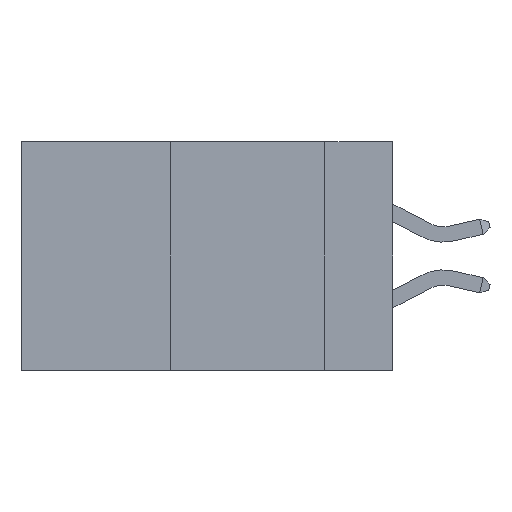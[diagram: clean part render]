
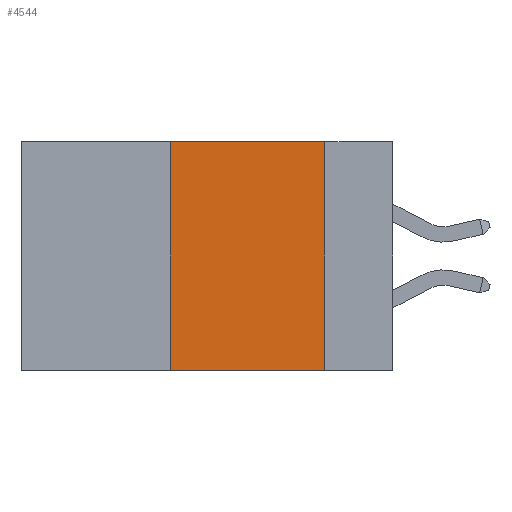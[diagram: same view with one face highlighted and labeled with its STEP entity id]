
A CAD part, left-side view. The second image highlights one B-rep face of the part: STEP entity #4544.
In plain terms, the highlighted planar face has unit normal (-1, 0, 0).
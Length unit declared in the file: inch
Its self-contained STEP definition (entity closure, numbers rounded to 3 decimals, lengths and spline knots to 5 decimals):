
#792 = DIRECTION ( 'NONE',  ( 0., 0., -1. ) ) ;
#850 = CARTESIAN_POINT ( 'NONE',  ( 0., 0.6, -0.37 ) ) ;
#1482 = CARTESIAN_POINT ( 'NONE',  ( 0., 0.6, 0. ) ) ;
#2125 = LINE ( 'NONE', #850, #16871 ) ;
#2255 = FACE_OUTER_BOUND ( 'NONE', #17594, .T. ) ;
#3643 = CARTESIAN_POINT ( 'NONE',  ( 0., 0.36, -0.37 ) ) ;
#4544 = ADVANCED_FACE ( 'NONE', ( #2255 ), #6492, .F. ) ;
#4695 = DIRECTION ( 'NONE',  ( 0., -1., 0. ) ) ;
#5399 = LINE ( 'NONE', #20824, #24518 ) ;
#5558 = VERTEX_POINT ( 'NONE', #3643 ) ;
#6116 = EDGE_CURVE ( 'NONE', #16704, #19668, #18142, .T. ) ;
#6232 = ORIENTED_EDGE ( 'NONE', *, *, #14198, .F. ) ;
#6492 = PLANE ( 'NONE',  #20774 ) ;
#6601 = CARTESIAN_POINT ( 'NONE',  ( 0., 0.11, 0. ) ) ;
#7314 = VECTOR ( 'NONE', #20564, 39.37008 ) ;
#7437 = DIRECTION ( 'NONE',  ( 0., 0., -1. ) ) ;
#9028 = EDGE_CURVE ( 'NONE', #5558, #19866, #2125, .T. ) ;
#10839 = CARTESIAN_POINT ( 'NONE',  ( 0., 0.36, 0. ) ) ;
#11573 = EDGE_CURVE ( 'NONE', #5558, #16704, #22942, .T. ) ;
#12264 = VECTOR ( 'NONE', #14738, 39.37008 ) ;
#12321 = DIRECTION ( 'NONE',  ( 1., 0., 0. ) ) ;
#14198 = EDGE_CURVE ( 'NONE', #19668, #19866, #5399, .T. ) ;
#14738 = DIRECTION ( 'NONE',  ( 0., 0., 1. ) ) ;
#15759 = CARTESIAN_POINT ( 'NONE',  ( 0., 0.36, 0. ) ) ;
#16704 = VERTEX_POINT ( 'NONE', #15759 ) ;
#16854 = CARTESIAN_POINT ( 'NONE',  ( 0., 0.11, -0.37 ) ) ;
#16871 = VECTOR ( 'NONE', #4695, 39.37008 ) ;
#17594 = EDGE_LOOP ( 'NONE', ( #6232, #22104, #22676, #18284 ) ) ;
#18142 = LINE ( 'NONE', #1482, #7314 ) ;
#18284 = ORIENTED_EDGE ( 'NONE', *, *, #9028, .T. ) ;
#19668 = VERTEX_POINT ( 'NONE', #6601 ) ;
#19866 = VERTEX_POINT ( 'NONE', #16854 ) ;
#20564 = DIRECTION ( 'NONE',  ( 0., -1., 0. ) ) ;
#20774 = AXIS2_PLACEMENT_3D ( 'NONE', #23677, #12321, #792 ) ;
#20824 = CARTESIAN_POINT ( 'NONE',  ( 0., 0.11, 0. ) ) ;
#22104 = ORIENTED_EDGE ( 'NONE', *, *, #6116, .F. ) ;
#22676 = ORIENTED_EDGE ( 'NONE', *, *, #11573, .F. ) ;
#22942 = LINE ( 'NONE', #10839, #12264 ) ;
#23677 = CARTESIAN_POINT ( 'NONE',  ( 0., 0.6, 0. ) ) ;
#24518 = VECTOR ( 'NONE', #7437, 39.37008 ) ;
